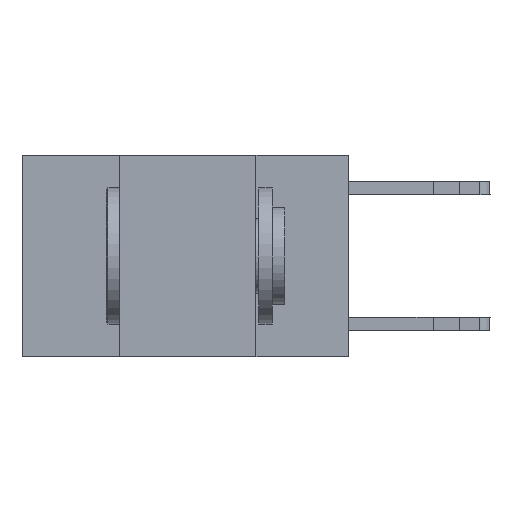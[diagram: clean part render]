
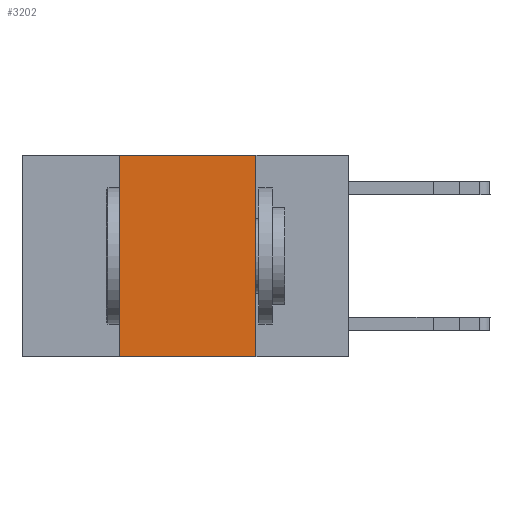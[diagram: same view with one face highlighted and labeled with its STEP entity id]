
A CAD part, left-side view. The second image highlights one B-rep face of the part: STEP entity #3202.
In plain terms, the highlighted planar face has unit normal (-1, 0, 0).
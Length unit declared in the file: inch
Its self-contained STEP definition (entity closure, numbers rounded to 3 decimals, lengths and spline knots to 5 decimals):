
#40 = LINE ( 'NONE', #11041, #3023 ) ;
#1463 = EDGE_CURVE ( 'NONE', #4663, #3688, #3561, .T. ) ;
#1938 = ORIENTED_EDGE ( 'NONE', *, *, #1463, .F. ) ;
#3023 = VECTOR ( 'NONE', #12973, 39.37008 ) ;
#3202 = ADVANCED_FACE ( 'NONE', ( #5112 ), #10898, .F. ) ;
#3561 = LINE ( 'NONE', #10919, #23472 ) ;
#3688 = VERTEX_POINT ( 'NONE', #23606 ) ;
#3854 = ORIENTED_EDGE ( 'NONE', *, *, #20340, .F. ) ;
#4663 = VERTEX_POINT ( 'NONE', #18770 ) ;
#5112 = FACE_OUTER_BOUND ( 'NONE', #6290, .T. ) ;
#5371 = DIRECTION ( 'NONE',  ( 0., -1., 0. ) ) ;
#5389 = EDGE_CURVE ( 'NONE', #4663, #19898, #40, .T. ) ;
#6290 = EDGE_LOOP ( 'NONE', ( #20085, #3854, #1938, #11063 ) ) ;
#6827 = CARTESIAN_POINT ( 'NONE',  ( 0., 0.6, 0. ) ) ;
#6913 = DIRECTION ( 'NONE',  ( 0., 0., -1. ) ) ;
#7270 = EDGE_CURVE ( 'NONE', #12890, #19898, #14210, .T. ) ;
#9630 = CARTESIAN_POINT ( 'NONE',  ( 0., 0.17, -0.37 ) ) ;
#10898 = PLANE ( 'NONE',  #20350 ) ;
#10919 = CARTESIAN_POINT ( 'NONE',  ( 0., 0.42, 0. ) ) ;
#11041 = CARTESIAN_POINT ( 'NONE',  ( 0., 0.6, -0.37 ) ) ;
#11063 = ORIENTED_EDGE ( 'NONE', *, *, #5389, .T. ) ;
#12596 = CARTESIAN_POINT ( 'NONE',  ( 0., 0.6, 0. ) ) ;
#12890 = VERTEX_POINT ( 'NONE', #18676 ) ;
#12973 = DIRECTION ( 'NONE',  ( 0., -1., 0. ) ) ;
#14099 = CARTESIAN_POINT ( 'NONE',  ( 0., 0.17, 0. ) ) ;
#14210 = LINE ( 'NONE', #14099, #19496 ) ;
#14677 = DIRECTION ( 'NONE',  ( 0., 0., 1. ) ) ;
#16347 = DIRECTION ( 'NONE',  ( 1., 0., 0. ) ) ;
#18676 = CARTESIAN_POINT ( 'NONE',  ( 0., 0.17, 0. ) ) ;
#18770 = CARTESIAN_POINT ( 'NONE',  ( 0., 0.42, -0.37 ) ) ;
#19496 = VECTOR ( 'NONE', #21473, 39.37008 ) ;
#19898 = VERTEX_POINT ( 'NONE', #9630 ) ;
#20085 = ORIENTED_EDGE ( 'NONE', *, *, #7270, .F. ) ;
#20340 = EDGE_CURVE ( 'NONE', #3688, #12890, #21950, .T. ) ;
#20350 = AXIS2_PLACEMENT_3D ( 'NONE', #12596, #16347, #6913 ) ;
#21198 = VECTOR ( 'NONE', #5371, 39.37008 ) ;
#21473 = DIRECTION ( 'NONE',  ( 0., 0., -1. ) ) ;
#21950 = LINE ( 'NONE', #6827, #21198 ) ;
#23472 = VECTOR ( 'NONE', #14677, 39.37008 ) ;
#23606 = CARTESIAN_POINT ( 'NONE',  ( 0., 0.42, 0. ) ) ;
